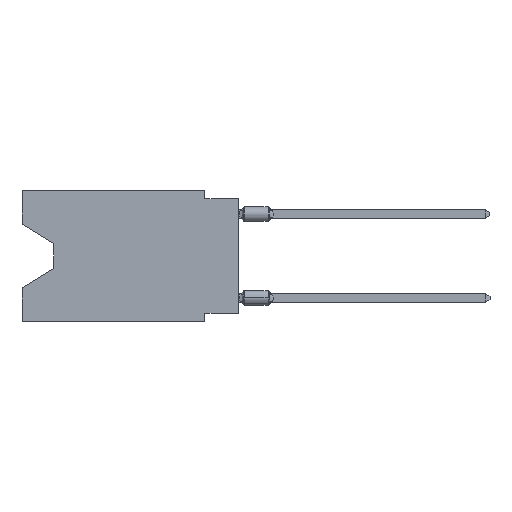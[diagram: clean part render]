
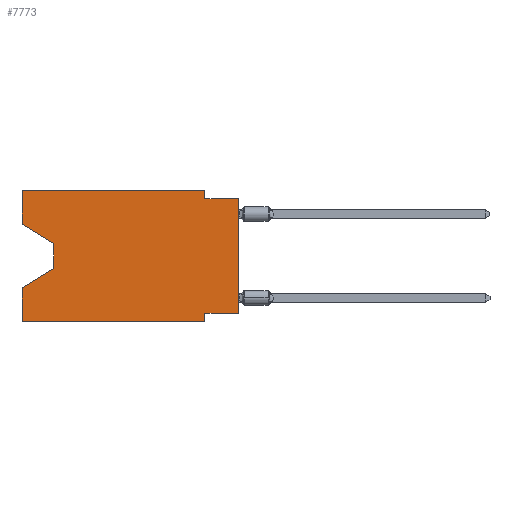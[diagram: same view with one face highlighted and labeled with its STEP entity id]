
A CAD part, left-side view. The second image highlights one B-rep face of the part: STEP entity #7773.
In plain terms, the highlighted planar face has unit normal (-1, 0, 0).
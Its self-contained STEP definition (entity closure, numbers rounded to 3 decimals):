
#5 = DIRECTION ( 'NONE',  ( 0., 0., 1. ) ) ;
#285 = ORIENTED_EDGE ( 'NONE', *, *, #11530, .T. ) ;
#358 = LINE ( 'NONE', #6611, #11763 ) ;
#455 = VECTOR ( 'NONE', #4656, 1000. ) ;
#467 = ORIENTED_EDGE ( 'NONE', *, *, #3022, .F. ) ;
#505 = LINE ( 'NONE', #7550, #455 ) ;
#1290 = DIRECTION ( 'NONE',  ( 0., 0., -1. ) ) ;
#1520 = CARTESIAN_POINT ( 'NONE',  ( 0., 0., 0. ) ) ;
#1547 = DIRECTION ( 'NONE',  ( 0., 0., -1. ) ) ;
#1638 = ORIENTED_EDGE ( 'NONE', *, *, #7017, .F. ) ;
#1750 = EDGE_CURVE ( 'NONE', #5989, #12811, #358, .T. ) ;
#1880 = CARTESIAN_POINT ( 'NONE',  ( 0., 0., -9.271 ) ) ;
#2005 = VECTOR ( 'NONE', #8193, 1000. ) ;
#2497 = VERTEX_POINT ( 'NONE', #7239 ) ;
#2603 = EDGE_CURVE ( 'NONE', #8655, #12811, #4402, .T. ) ;
#2705 = CARTESIAN_POINT ( 'NONE',  ( 0., 0., -0.635 ) ) ;
#2751 = CARTESIAN_POINT ( 'NONE',  ( 0., 16.383, 0. ) ) ;
#3009 = CARTESIAN_POINT ( 'NONE',  ( 0., 2.54, -9.271 ) ) ;
#3022 = EDGE_CURVE ( 'NONE', #6248, #9881, #505, .T. ) ;
#3154 = LINE ( 'NONE', #4206, #11386 ) ;
#3236 = CARTESIAN_POINT ( 'NONE',  ( 0., 16.383, -9.906 ) ) ;
#3427 = EDGE_CURVE ( 'NONE', #4452, #8223, #10874, .T. ) ;
#3501 = EDGE_CURVE ( 'NONE', #3769, #12431, #9097, .T. ) ;
#3516 = EDGE_CURVE ( 'NONE', #4158, #6248, #3154, .T. ) ;
#3769 = VERTEX_POINT ( 'NONE', #7708 ) ;
#3812 = VECTOR ( 'NONE', #5262, 1000. ) ;
#3978 = EDGE_CURVE ( 'NONE', #4158, #11669, #9215, .T. ) ;
#4037 = VECTOR ( 'NONE', #11191, 1000. ) ;
#4044 = CARTESIAN_POINT ( 'NONE',  ( 0., 16.383, -7.36 ) ) ;
#4119 = EDGE_CURVE ( 'NONE', #9881, #4452, #7296, .T. ) ;
#4158 = VERTEX_POINT ( 'NONE', #12475 ) ;
#4206 = CARTESIAN_POINT ( 'NONE',  ( 0., 16.383, 0. ) ) ;
#4336 = DIRECTION ( 'NONE',  ( 0., 0., -1. ) ) ;
#4379 = LINE ( 'NONE', #7210, #2005 ) ;
#4402 = LINE ( 'NONE', #11373, #3812 ) ;
#4452 = VERTEX_POINT ( 'NONE', #9259 ) ;
#4466 = EDGE_CURVE ( 'NONE', #11669, #3769, #4379, .T. ) ;
#4582 = PLANE ( 'NONE',  #11263 ) ;
#4656 = DIRECTION ( 'NONE',  ( 0., -1., 0. ) ) ;
#5185 = ORIENTED_EDGE ( 'NONE', *, *, #7560, .F. ) ;
#5262 = DIRECTION ( 'NONE',  ( 0., -1., 0. ) ) ;
#5265 = CARTESIAN_POINT ( 'NONE',  ( 0., 13.97, -5.893 ) ) ;
#5498 = CARTESIAN_POINT ( 'NONE',  ( 0., 16.383, 0. ) ) ;
#5532 = VECTOR ( 'NONE', #8570, 1000. ) ;
#5728 = LINE ( 'NONE', #1520, #5532 ) ;
#5735 = ORIENTED_EDGE ( 'NONE', *, *, #3427, .F. ) ;
#5901 = DIRECTION ( 'NONE',  ( 0., 1., 0. ) ) ;
#5925 = DIRECTION ( 'NONE',  ( 0., -0.855, -0.519 ) ) ;
#5989 = VERTEX_POINT ( 'NONE', #3009 ) ;
#6248 = VERTEX_POINT ( 'NONE', #10903 ) ;
#6495 = ORIENTED_EDGE ( 'NONE', *, *, #3516, .F. ) ;
#6551 = FACE_OUTER_BOUND ( 'NONE', #12386, .T. ) ;
#6611 = CARTESIAN_POINT ( 'NONE',  ( 0., 2.54, -9.906 ) ) ;
#6720 = DIRECTION ( 'NONE',  ( 0., -1., 0. ) ) ;
#6916 = CARTESIAN_POINT ( 'NONE',  ( 0., 2.54, 0. ) ) ;
#7017 = EDGE_CURVE ( 'NONE', #8655, #12431, #11771, .T. ) ;
#7203 = VECTOR ( 'NONE', #5925, 1000. ) ;
#7210 = CARTESIAN_POINT ( 'NONE',  ( 0., 13.97, -4.013 ) ) ;
#7239 = CARTESIAN_POINT ( 'NONE',  ( 0., 0., -9.271 ) ) ;
#7258 = VECTOR ( 'NONE', #7903, 1000. ) ;
#7296 = LINE ( 'NONE', #9273, #8265 ) ;
#7550 = CARTESIAN_POINT ( 'NONE',  ( 0., 16.383, 0. ) ) ;
#7560 = EDGE_CURVE ( 'NONE', #2497, #5989, #12796, .T. ) ;
#7569 = ORIENTED_EDGE ( 'NONE', *, *, #4119, .F. ) ;
#7708 = CARTESIAN_POINT ( 'NONE',  ( 0., 13.97, -5.893 ) ) ;
#7773 = ADVANCED_FACE ( 'NONE', ( #6551 ), #4582, .F. ) ;
#7903 = DIRECTION ( 'NONE',  ( 0., 0., 1. ) ) ;
#8113 = ORIENTED_EDGE ( 'NONE', *, *, #4466, .T. ) ;
#8193 = DIRECTION ( 'NONE',  ( 0., 0., -1. ) ) ;
#8223 = VERTEX_POINT ( 'NONE', #11527 ) ;
#8265 = VECTOR ( 'NONE', #4336, 1000. ) ;
#8400 = DIRECTION ( 'NONE',  ( 1., 0., 0. ) ) ;
#8570 = DIRECTION ( 'NONE',  ( 0., 0., 1. ) ) ;
#8655 = VERTEX_POINT ( 'NONE', #3236 ) ;
#8670 = VECTOR ( 'NONE', #6720, 1000. ) ;
#8755 = ORIENTED_EDGE ( 'NONE', *, *, #2603, .T. ) ;
#8927 = ORIENTED_EDGE ( 'NONE', *, *, #1750, .F. ) ;
#9018 = CARTESIAN_POINT ( 'NONE',  ( 0., 16.383, -2.546 ) ) ;
#9097 = LINE ( 'NONE', #5265, #4037 ) ;
#9215 = LINE ( 'NONE', #9018, #7203 ) ;
#9259 = CARTESIAN_POINT ( 'NONE',  ( 0., 2.54, -0.635 ) ) ;
#9273 = CARTESIAN_POINT ( 'NONE',  ( 0., 2.54, 0. ) ) ;
#9881 = VERTEX_POINT ( 'NONE', #6916 ) ;
#10212 = VECTOR ( 'NONE', #5901, 1000. ) ;
#10256 = CARTESIAN_POINT ( 'NONE',  ( 0., 13.97, -4.013 ) ) ;
#10874 = LINE ( 'NONE', #2705, #8670 ) ;
#10903 = CARTESIAN_POINT ( 'NONE',  ( 0., 16.383, 0. ) ) ;
#10935 = CARTESIAN_POINT ( 'NONE',  ( 0., 2.54, -9.906 ) ) ;
#11191 = DIRECTION ( 'NONE',  ( 0., 0.855, -0.519 ) ) ;
#11235 = ORIENTED_EDGE ( 'NONE', *, *, #3978, .T. ) ;
#11263 = AXIS2_PLACEMENT_3D ( 'NONE', #5498, #8400, #1290 ) ;
#11373 = CARTESIAN_POINT ( 'NONE',  ( 0., 16.383, -9.906 ) ) ;
#11386 = VECTOR ( 'NONE', #5, 1000. ) ;
#11527 = CARTESIAN_POINT ( 'NONE',  ( 0., 0., -0.635 ) ) ;
#11530 = EDGE_CURVE ( 'NONE', #2497, #8223, #5728, .T. ) ;
#11669 = VERTEX_POINT ( 'NONE', #10256 ) ;
#11763 = VECTOR ( 'NONE', #1547, 1000. ) ;
#11771 = LINE ( 'NONE', #2751, #7258 ) ;
#12386 = EDGE_LOOP ( 'NONE', ( #11235, #8113, #12917, #1638, #8755, #8927, #5185, #285, #5735, #7569, #467, #6495 ) ) ;
#12431 = VERTEX_POINT ( 'NONE', #4044 ) ;
#12475 = CARTESIAN_POINT ( 'NONE',  ( 0., 16.383, -2.546 ) ) ;
#12796 = LINE ( 'NONE', #1880, #10212 ) ;
#12811 = VERTEX_POINT ( 'NONE', #10935 ) ;
#12917 = ORIENTED_EDGE ( 'NONE', *, *, #3501, .T. ) ;
